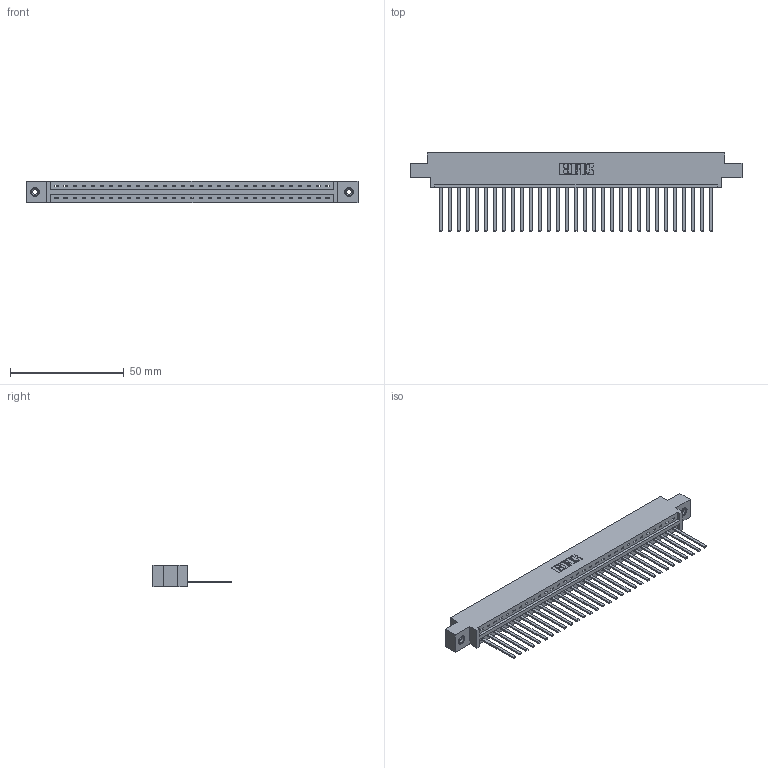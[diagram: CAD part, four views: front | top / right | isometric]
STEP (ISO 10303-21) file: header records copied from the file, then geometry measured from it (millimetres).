
FILE_DESCRIPTION (( 'STEP AP203' ), '1' );
FILE_NAME ('337-031-544-608.STEP', '2018-08-07T03:53:34', ( '' ), ( '' ), 'SwSTEP 2.0', 'SolidWorks 2016', '' );
FILE_SCHEMA (( 'CONFIG_CONTROL_DESIGN' ));
Length unit declared in the file: inch
Products named in the file (4): 337 Part_0.170 Offset - 0.156 Dia-TI; 345-292-001_345-293-144; 345-250-001_345-250-003-102; 337-031-544-608
Assembly tree (34 placements, depth 2):
  337-031-544-608
    337 Part_0.170 Offset - 0.156 Dia-TI
    345-292-001_345-293-144  x31
    345-250-001_345-250-003-102  x2
Bounding box: 145.85 x 34.3 x 9.4 mm (x, y, z)
Volume: 15255.7 mm3; surface area: 17010.6 mm2
Topology: 34 solids, 34 shells, 1914 faces, 5729 edges, 3770 vertices
Faces by surface type: plane 1408, cylinder 490, cone 12, torus 4
Entity records: 25600 total; most frequent: CARTESIAN_POINT 4438, ORIENTED_EDGE 4398, DIRECTION 3787, EDGE_CURVE 2199, LINE 2055, VECTOR 2055, VERTEX_POINT 1460, AXIS2_PLACEMENT_3D 866
